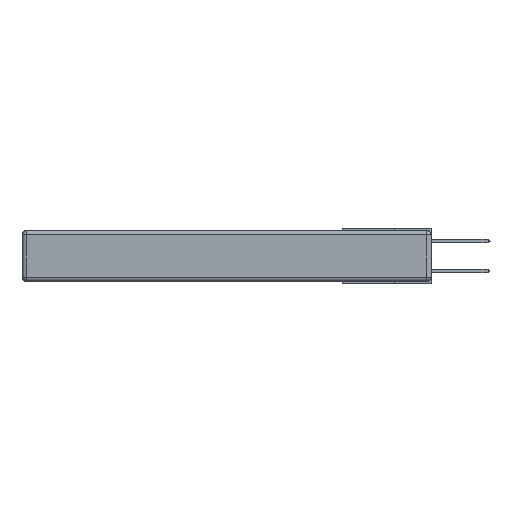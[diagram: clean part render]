
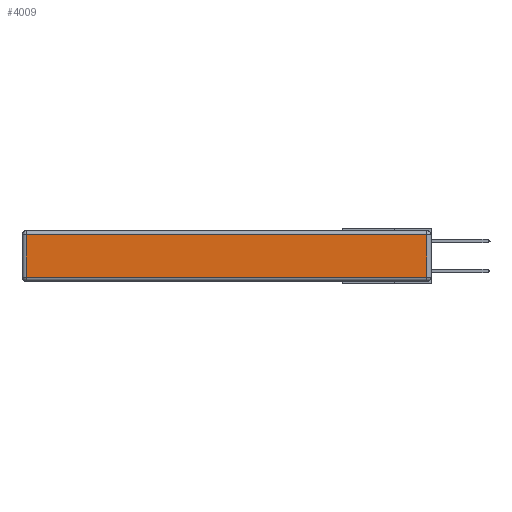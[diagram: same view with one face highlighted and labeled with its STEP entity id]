
A CAD part, left-side view. The second image highlights one B-rep face of the part: STEP entity #4009.
In plain terms, the highlighted planar face has unit normal (-1, 0, 0).
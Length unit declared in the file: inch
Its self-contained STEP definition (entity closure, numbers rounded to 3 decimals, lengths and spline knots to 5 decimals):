
#375 = CARTESIAN_POINT ( 'NONE',  ( 0., 2.75, -0.03 ) ) ;
#1491 = ORIENTED_EDGE ( 'NONE', *, *, #12877, .T. ) ;
#2368 = ORIENTED_EDGE ( 'NONE', *, *, #5818, .T. ) ;
#2718 = DIRECTION ( 'NONE',  ( 0., 0., 1. ) ) ;
#3147 = VECTOR ( 'NONE', #9444, 39.37008 ) ;
#3377 = VECTOR ( 'NONE', #13841, 39.37008 ) ;
#4009 = ADVANCED_FACE ( 'NONE', ( #12083 ), #14668, .T. ) ;
#4214 = ORIENTED_EDGE ( 'NONE', *, *, #14627, .T. ) ;
#5698 = CARTESIAN_POINT ( 'NONE',  ( 0., 2.72, -0.313 ) ) ;
#5818 = EDGE_CURVE ( 'NONE', #15337, #6950, #7615, .T. ) ;
#6248 = DIRECTION ( 'NONE',  ( 0., 0., 1. ) ) ;
#6324 = ORIENTED_EDGE ( 'NONE', *, *, #17170, .T. ) ;
#6950 = VERTEX_POINT ( 'NONE', #17900 ) ;
#7067 = LINE ( 'NONE', #375, #3377 ) ;
#7615 = LINE ( 'NONE', #17808, #3147 ) ;
#7645 = EDGE_LOOP ( 'NONE', ( #2368, #1491, #4214, #6324 ) ) ;
#7648 = VECTOR ( 'NONE', #6248, 39.37008 ) ;
#7894 = VERTEX_POINT ( 'NONE', #18985 ) ;
#8032 = AXIS2_PLACEMENT_3D ( 'NONE', #17635, #19386, #2718 ) ;
#8277 = CARTESIAN_POINT ( 'NONE',  ( 0., 0.03, -0.343 ) ) ;
#9402 = CARTESIAN_POINT ( 'NONE',  ( 0., 2.72, -0.343 ) ) ;
#9444 = DIRECTION ( 'NONE',  ( 0., -1., 0. ) ) ;
#9799 = LINE ( 'NONE', #8277, #7648 ) ;
#12083 = FACE_OUTER_BOUND ( 'NONE', #7645, .T. ) ;
#12877 = EDGE_CURVE ( 'NONE', #6950, #7894, #9799, .T. ) ;
#13841 = DIRECTION ( 'NONE',  ( 0., 1., 0. ) ) ;
#14627 = EDGE_CURVE ( 'NONE', #7894, #18785, #7067, .T. ) ;
#14668 = PLANE ( 'NONE',  #8032 ) ;
#14882 = LINE ( 'NONE', #9402, #19302 ) ;
#15337 = VERTEX_POINT ( 'NONE', #5698 ) ;
#16079 = CARTESIAN_POINT ( 'NONE',  ( 0., 2.72, -0.03 ) ) ;
#16191 = DIRECTION ( 'NONE',  ( 0., 0., -1. ) ) ;
#17170 = EDGE_CURVE ( 'NONE', #18785, #15337, #14882, .T. ) ;
#17635 = CARTESIAN_POINT ( 'NONE',  ( 0., 0., -0.343 ) ) ;
#17808 = CARTESIAN_POINT ( 'NONE',  ( 0., 0., -0.313 ) ) ;
#17900 = CARTESIAN_POINT ( 'NONE',  ( 0., 0.03, -0.313 ) ) ;
#18785 = VERTEX_POINT ( 'NONE', #16079 ) ;
#18985 = CARTESIAN_POINT ( 'NONE',  ( 0., 0.03, -0.03 ) ) ;
#19302 = VECTOR ( 'NONE', #16191, 39.37008 ) ;
#19386 = DIRECTION ( 'NONE',  ( -1., 0., 0. ) ) ;
